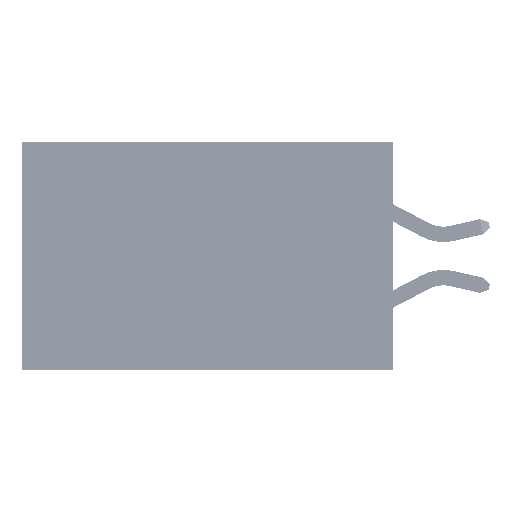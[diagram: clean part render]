
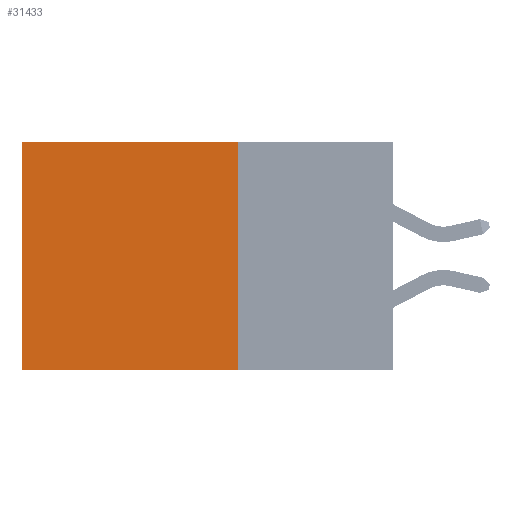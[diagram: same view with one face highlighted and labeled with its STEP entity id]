
A CAD part, left-side view. The second image highlights one B-rep face of the part: STEP entity #31433.
In plain terms, the highlighted planar face has unit normal (-1, 0, 0).
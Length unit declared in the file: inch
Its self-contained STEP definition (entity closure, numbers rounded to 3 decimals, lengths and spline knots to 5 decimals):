
#1024 = ORIENTED_EDGE ( 'NONE', *, *, #6457, .F. ) ;
#1590 = CARTESIAN_POINT ( 'NONE',  ( 0.2875, 0.25, 0. ) ) ;
#1714 = EDGE_CURVE ( 'NONE', #33359, #42113, #42424, .T. ) ;
#2530 = CARTESIAN_POINT ( 'NONE',  ( 0.2875, 0.6, 0. ) ) ;
#3924 = VECTOR ( 'NONE', #22259, 39.37008 ) ;
#4231 = CARTESIAN_POINT ( 'NONE',  ( 0.2875, 0.25, 0. ) ) ;
#4569 = EDGE_CURVE ( 'NONE', #33359, #15725, #11873, .T. ) ;
#6457 = EDGE_CURVE ( 'NONE', #15725, #11330, #25261, .T. ) ;
#8893 = ORIENTED_EDGE ( 'NONE', *, *, #1714, .T. ) ;
#9293 = CARTESIAN_POINT ( 'NONE',  ( 0.2875, 0.25, -0.37 ) ) ;
#11330 = VERTEX_POINT ( 'NONE', #18457 ) ;
#11873 = LINE ( 'NONE', #4231, #25445 ) ;
#12506 = DIRECTION ( 'NONE',  ( 0., 0., -1. ) ) ;
#12911 = DIRECTION ( 'NONE',  ( 0., 0., -1. ) ) ;
#14633 = CARTESIAN_POINT ( 'NONE',  ( 0.2875, 0.25, -0.37 ) ) ;
#15262 = CARTESIAN_POINT ( 'NONE',  ( 0.2875, 0.25, 0. ) ) ;
#15725 = VERTEX_POINT ( 'NONE', #9293 ) ;
#17426 = LINE ( 'NONE', #29787, #39679 ) ;
#18457 = CARTESIAN_POINT ( 'NONE',  ( 0.2875, 0.6, -0.37 ) ) ;
#20026 = CARTESIAN_POINT ( 'NONE',  ( 0.2875, 0.25, 0. ) ) ;
#20169 = DIRECTION ( 'NONE',  ( 1., 0., 0. ) ) ;
#20783 = FACE_OUTER_BOUND ( 'NONE', #26606, .T. ) ;
#20923 = VECTOR ( 'NONE', #21814, 39.37008 ) ;
#21814 = DIRECTION ( 'NONE',  ( 0., 1., 0. ) ) ;
#22259 = DIRECTION ( 'NONE',  ( 0., 1., 0. ) ) ;
#25261 = LINE ( 'NONE', #14633, #20923 ) ;
#25445 = VECTOR ( 'NONE', #29098, 39.37008 ) ;
#26606 = EDGE_LOOP ( 'NONE', ( #44277, #1024, #42697, #8893 ) ) ;
#29098 = DIRECTION ( 'NONE',  ( 0., 0., -1. ) ) ;
#29787 = CARTESIAN_POINT ( 'NONE',  ( 0.2875, 0.6, 0. ) ) ;
#30552 = AXIS2_PLACEMENT_3D ( 'NONE', #20026, #20169, #12911 ) ;
#31433 = ADVANCED_FACE ( 'NONE', ( #20783 ), #33385, .F. ) ;
#33359 = VERTEX_POINT ( 'NONE', #1590 ) ;
#33385 = PLANE ( 'NONE',  #30552 ) ;
#39679 = VECTOR ( 'NONE', #12506, 39.37008 ) ;
#42113 = VERTEX_POINT ( 'NONE', #2530 ) ;
#42424 = LINE ( 'NONE', #15262, #3924 ) ;
#42593 = EDGE_CURVE ( 'NONE', #42113, #11330, #17426, .T. ) ;
#42697 = ORIENTED_EDGE ( 'NONE', *, *, #4569, .F. ) ;
#44277 = ORIENTED_EDGE ( 'NONE', *, *, #42593, .T. ) ;
